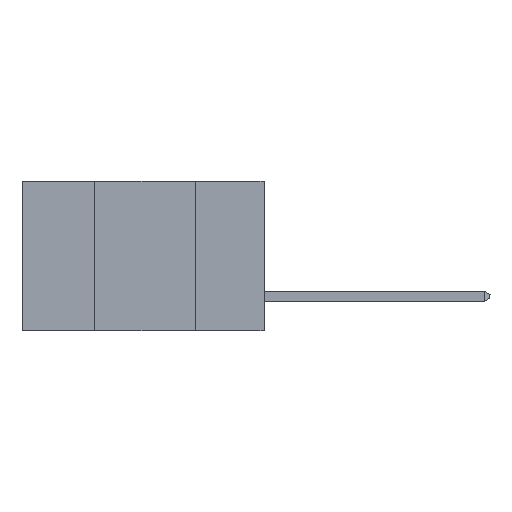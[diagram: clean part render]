
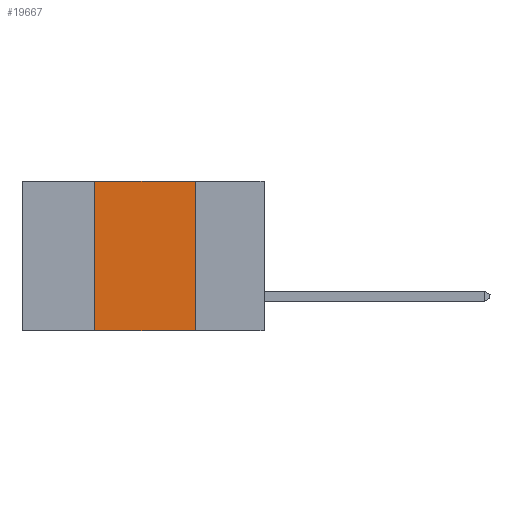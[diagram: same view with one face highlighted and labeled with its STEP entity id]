
A CAD part, left-side view. The second image highlights one B-rep face of the part: STEP entity #19667.
In plain terms, the highlighted planar face has unit normal (-1, 0, 0).
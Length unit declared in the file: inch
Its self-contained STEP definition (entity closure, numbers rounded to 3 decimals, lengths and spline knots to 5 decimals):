
#1333 = DIRECTION ( 'NONE',  ( 0., 0., -1. ) ) ;
#2829 = VECTOR ( 'NONE', #1333, 39.37008 ) ;
#3403 = DIRECTION ( 'NONE',  ( 1., 0., 0. ) ) ;
#4303 = CARTESIAN_POINT ( 'NONE',  ( 0., 0.6, 0. ) ) ;
#5869 = DIRECTION ( 'NONE',  ( 0., 0., -1. ) ) ;
#5894 = LINE ( 'NONE', #6136, #2829 ) ;
#6136 = CARTESIAN_POINT ( 'NONE',  ( 0., 0.17, 0. ) ) ;
#7761 = CARTESIAN_POINT ( 'NONE',  ( 0., 0.42, 0. ) ) ;
#7823 = EDGE_CURVE ( 'NONE', #15451, #23221, #21374, .T. ) ;
#8062 = CARTESIAN_POINT ( 'NONE',  ( 0., 0.17, 0. ) ) ;
#10039 = VECTOR ( 'NONE', #22093, 39.37008 ) ;
#10854 = VERTEX_POINT ( 'NONE', #7761 ) ;
#11951 = CARTESIAN_POINT ( 'NONE',  ( 0., 0.42, -0.37 ) ) ;
#12144 = LINE ( 'NONE', #4303, #18328 ) ;
#13339 = EDGE_CURVE ( 'NONE', #15451, #10854, #25468, .T. ) ;
#13632 = EDGE_LOOP ( 'NONE', ( #26853, #24291, #30021, #13779 ) ) ;
#13779 = ORIENTED_EDGE ( 'NONE', *, *, #7823, .T. ) ;
#13785 = DIRECTION ( 'NONE',  ( 0., -1., 0. ) ) ;
#13797 = FACE_OUTER_BOUND ( 'NONE', #13632, .T. ) ;
#14235 = CARTESIAN_POINT ( 'NONE',  ( 0., 0.6, -0.37 ) ) ;
#15451 = VERTEX_POINT ( 'NONE', #11951 ) ;
#17058 = EDGE_CURVE ( 'NONE', #10854, #28816, #12144, .T. ) ;
#17701 = AXIS2_PLACEMENT_3D ( 'NONE', #18036, #3403, #5869 ) ;
#18036 = CARTESIAN_POINT ( 'NONE',  ( 0., 0.6, 0. ) ) ;
#18328 = VECTOR ( 'NONE', #21484, 39.37008 ) ;
#19667 = ADVANCED_FACE ( 'NONE', ( #13797 ), #30608, .F. ) ;
#19936 = CARTESIAN_POINT ( 'NONE',  ( 0., 0.42, 0. ) ) ;
#21374 = LINE ( 'NONE', #14235, #22905 ) ;
#21484 = DIRECTION ( 'NONE',  ( 0., -1., 0. ) ) ;
#22093 = DIRECTION ( 'NONE',  ( 0., 0., 1. ) ) ;
#22905 = VECTOR ( 'NONE', #13785, 39.37008 ) ;
#23221 = VERTEX_POINT ( 'NONE', #26882 ) ;
#24291 = ORIENTED_EDGE ( 'NONE', *, *, #17058, .F. ) ;
#25468 = LINE ( 'NONE', #19936, #10039 ) ;
#26853 = ORIENTED_EDGE ( 'NONE', *, *, #31839, .F. ) ;
#26882 = CARTESIAN_POINT ( 'NONE',  ( 0., 0.17, -0.37 ) ) ;
#28816 = VERTEX_POINT ( 'NONE', #8062 ) ;
#30021 = ORIENTED_EDGE ( 'NONE', *, *, #13339, .F. ) ;
#30608 = PLANE ( 'NONE',  #17701 ) ;
#31839 = EDGE_CURVE ( 'NONE', #28816, #23221, #5894, .T. ) ;
